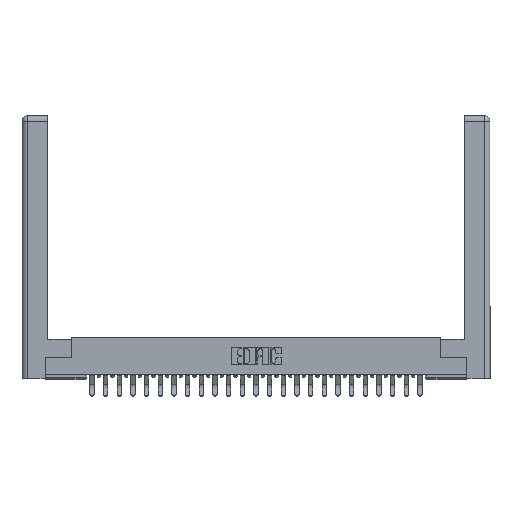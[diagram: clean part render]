
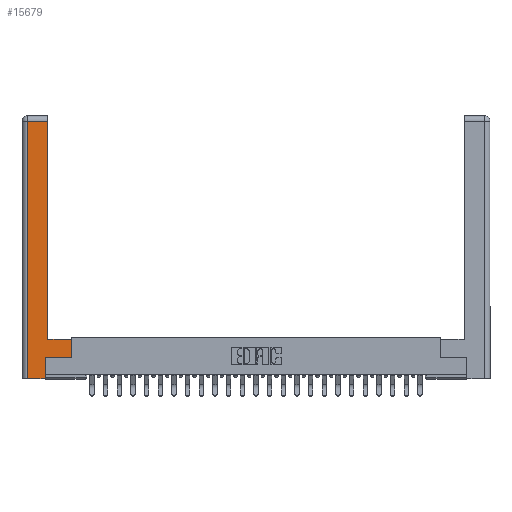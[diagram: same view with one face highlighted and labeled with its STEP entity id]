
A CAD part, top view. The second image highlights one B-rep face of the part: STEP entity #15679.
In plain terms, the highlighted planar face has unit normal (0, 0, 1).
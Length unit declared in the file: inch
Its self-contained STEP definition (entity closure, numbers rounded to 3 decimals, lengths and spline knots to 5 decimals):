
#32 = VERTEX_POINT ( 'NONE', #6247 ) ;
#362 = ORIENTED_EDGE ( 'NONE', *, *, #6598, .T. ) ;
#762 = ORIENTED_EDGE ( 'NONE', *, *, #1368, .T. ) ;
#813 = VECTOR ( 'NONE', #22988, 39.37008 ) ;
#1067 = CARTESIAN_POINT ( 'NONE',  ( 0.0615, 2.94, 0. ) ) ;
#1195 = EDGE_CURVE ( 'NONE', #22149, #3476, #24924, .T. ) ;
#1368 = EDGE_CURVE ( 'NONE', #10343, #32, #8884, .T. ) ;
#1702 = LINE ( 'NONE', #16020, #26895 ) ;
#1740 = EDGE_CURVE ( 'NONE', #14581, #11638, #12547, .T. ) ;
#2638 = DIRECTION ( 'NONE',  ( 0., 1., 0. ) ) ;
#3379 = CARTESIAN_POINT ( 'NONE',  ( 0.565, 0.245, 0. ) ) ;
#3476 = VERTEX_POINT ( 'NONE', #14285 ) ;
#4033 = VERTEX_POINT ( 'NONE', #18073 ) ;
#4740 = ORIENTED_EDGE ( 'NONE', *, *, #1740, .T. ) ;
#4810 = VECTOR ( 'NONE', #22265, 39.37008 ) ;
#5078 = CARTESIAN_POINT ( 'NONE',  ( 0.565, 0.45, 0. ) ) ;
#5153 = LINE ( 'NONE', #20446, #4810 ) ;
#5435 = DIRECTION ( 'NONE',  ( 0., 0., -1. ) ) ;
#5529 = CARTESIAN_POINT ( 'NONE',  ( 0., 0., 0. ) ) ;
#5947 = EDGE_CURVE ( 'NONE', #11638, #10343, #18862, .T. ) ;
#6165 = ORIENTED_EDGE ( 'NONE', *, *, #8451, .T. ) ;
#6247 = CARTESIAN_POINT ( 'NONE',  ( 0.295, 2.94, 0. ) ) ;
#6598 = EDGE_CURVE ( 'NONE', #14557, #4033, #22083, .T. ) ;
#7002 = CARTESIAN_POINT ( 'NONE',  ( 0.265, 0., 0. ) ) ;
#7032 = ORIENTED_EDGE ( 'NONE', *, *, #5947, .T. ) ;
#7182 = AXIS2_PLACEMENT_3D ( 'NONE', #5529, #5435, #7800 ) ;
#7800 = DIRECTION ( 'NONE',  ( -1., 0., 0. ) ) ;
#8369 = CARTESIAN_POINT ( 'NONE',  ( 0.295, 0.45, 0. ) ) ;
#8451 = EDGE_CURVE ( 'NONE', #32, #14557, #11216, .T. ) ;
#8884 = LINE ( 'NONE', #23313, #24269 ) ;
#9244 = CARTESIAN_POINT ( 'NONE',  ( 0.0615, 2.94, 0. ) ) ;
#10343 = VERTEX_POINT ( 'NONE', #17950 ) ;
#10666 = VECTOR ( 'NONE', #20755, 39.37008 ) ;
#10835 = DIRECTION ( 'NONE',  ( 0., 1., 0. ) ) ;
#11216 = LINE ( 'NONE', #1067, #11878 ) ;
#11638 = VERTEX_POINT ( 'NONE', #5078 ) ;
#11878 = VECTOR ( 'NONE', #20006, 39.37008 ) ;
#12547 = LINE ( 'NONE', #20756, #21359 ) ;
#13469 = EDGE_CURVE ( 'NONE', #4033, #22149, #5153, .T. ) ;
#13795 = EDGE_LOOP ( 'NONE', ( #762, #6165, #362, #19756, #15044, #22851, #4740, #7032 ) ) ;
#14285 = CARTESIAN_POINT ( 'NONE',  ( 0.265, 0.245, 0. ) ) ;
#14557 = VERTEX_POINT ( 'NONE', #9244 ) ;
#14581 = VERTEX_POINT ( 'NONE', #3379 ) ;
#15044 = ORIENTED_EDGE ( 'NONE', *, *, #1195, .T. ) ;
#15679 = ADVANCED_FACE ( 'NONE', ( #23652 ), #17966, .F. ) ;
#16020 = CARTESIAN_POINT ( 'NONE',  ( 0.565, 0.245, 0. ) ) ;
#16364 = CARTESIAN_POINT ( 'NONE',  ( 0.0615, 0., 0. ) ) ;
#17950 = CARTESIAN_POINT ( 'NONE',  ( 0.295, 0.45, 0. ) ) ;
#17966 = PLANE ( 'NONE',  #7182 ) ;
#18073 = CARTESIAN_POINT ( 'NONE',  ( 0.0615, 0., 0. ) ) ;
#18550 = EDGE_CURVE ( 'NONE', #3476, #14581, #1702, .T. ) ;
#18862 = LINE ( 'NONE', #8369, #813 ) ;
#19756 = ORIENTED_EDGE ( 'NONE', *, *, #13469, .T. ) ;
#20006 = DIRECTION ( 'NONE',  ( -1., 0., 0. ) ) ;
#20446 = CARTESIAN_POINT ( 'NONE',  ( 0.265, 0., 0. ) ) ;
#20755 = DIRECTION ( 'NONE',  ( 0., -1., 0. ) ) ;
#20756 = CARTESIAN_POINT ( 'NONE',  ( 0.565, 0.45, 0. ) ) ;
#21359 = VECTOR ( 'NONE', #24670, 39.37008 ) ;
#22083 = LINE ( 'NONE', #16364, #10666 ) ;
#22149 = VERTEX_POINT ( 'NONE', #7002 ) ;
#22229 = DIRECTION ( 'NONE',  ( 1., 0., 0. ) ) ;
#22265 = DIRECTION ( 'NONE',  ( 1., 0., 0. ) ) ;
#22851 = ORIENTED_EDGE ( 'NONE', *, *, #18550, .T. ) ;
#22988 = DIRECTION ( 'NONE',  ( -1., 0., 0. ) ) ;
#23313 = CARTESIAN_POINT ( 'NONE',  ( 0.295, 3., 0. ) ) ;
#23652 = FACE_OUTER_BOUND ( 'NONE', #13795, .T. ) ;
#24269 = VECTOR ( 'NONE', #10835, 39.37008 ) ;
#24670 = DIRECTION ( 'NONE',  ( 0., 1., 0. ) ) ;
#24924 = LINE ( 'NONE', #25873, #25933 ) ;
#25873 = CARTESIAN_POINT ( 'NONE',  ( 0.265, 0.245, 0. ) ) ;
#25933 = VECTOR ( 'NONE', #2638, 39.37008 ) ;
#26895 = VECTOR ( 'NONE', #22229, 39.37008 ) ;
